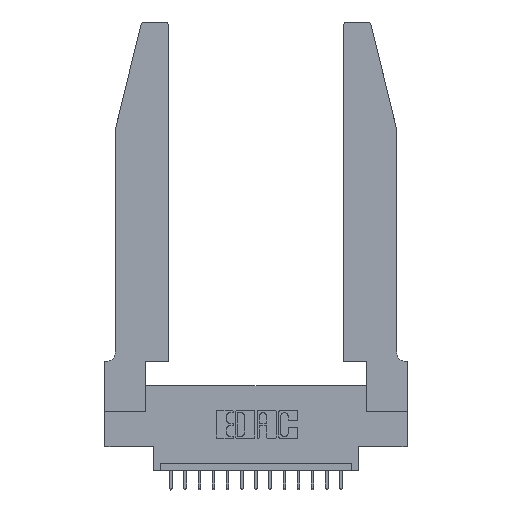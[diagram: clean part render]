
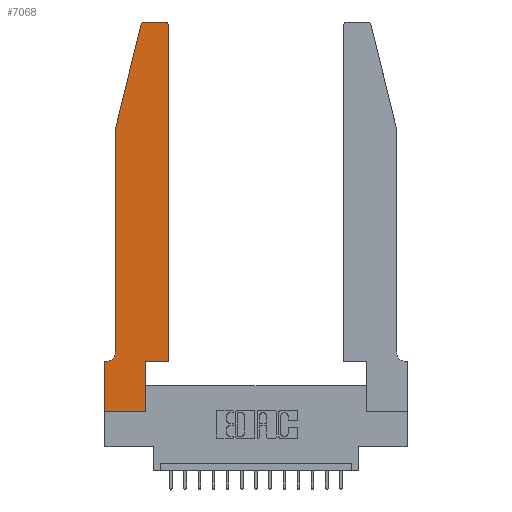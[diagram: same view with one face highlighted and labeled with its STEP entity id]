
A CAD part, top view. The second image highlights one B-rep face of the part: STEP entity #7068.
In plain terms, the highlighted planar face has unit normal (0, 0, 1).
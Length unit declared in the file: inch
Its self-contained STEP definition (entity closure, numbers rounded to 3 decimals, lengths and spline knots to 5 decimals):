
#320 = VERTEX_POINT ( 'NONE', #3296 ) ;
#523 = AXIS2_PLACEMENT_3D ( 'NONE', #9767, #8075, #13805 ) ;
#850 = VECTOR ( 'NONE', #7060, 39.37008 ) ;
#905 = VERTEX_POINT ( 'NONE', #1213 ) ;
#1090 = CIRCLE ( 'NONE', #15275, 0.03 ) ;
#1213 = CARTESIAN_POINT ( 'NONE',  ( 0.4205, 2.75, 0.37 ) ) ;
#1364 = CARTESIAN_POINT ( 'NONE',  ( 0.2865, 0.35, 0.37 ) ) ;
#1635 = VECTOR ( 'NONE', #4557, 39.37008 ) ;
#1688 = CARTESIAN_POINT ( 'NONE',  ( 0.4505, 0.35, 0.37 ) ) ;
#1705 = EDGE_CURVE ( 'NONE', #9627, #12850, #8957, .T. ) ;
#1714 = VERTEX_POINT ( 'NONE', #7247 ) ;
#1772 = DIRECTION ( 'NONE',  ( 0., 0., 1. ) ) ;
#1871 = EDGE_LOOP ( 'NONE', ( #9339, #7914, #3779, #16202, #6469, #6938, #16929, #7415, #16541, #7703, #12830, #9924 ) ) ;
#1991 = VERTEX_POINT ( 'NONE', #5051 ) ;
#2058 = CIRCLE ( 'NONE', #523, 0.07 ) ;
#2537 = DIRECTION ( 'NONE',  ( 0., 0., 1. ) ) ;
#3296 = CARTESIAN_POINT ( 'NONE',  ( 0.0755, 0.42, 0.37 ) ) ;
#3378 = EDGE_CURVE ( 'NONE', #17656, #9627, #1090, .T. ) ;
#3597 = CARTESIAN_POINT ( 'NONE',  ( 0., 0., 0.37 ) ) ;
#3779 = ORIENTED_EDGE ( 'NONE', *, *, #1705, .T. ) ;
#3914 = EDGE_CURVE ( 'NONE', #11699, #12863, #8164, .T. ) ;
#3939 = EDGE_CURVE ( 'NONE', #320, #15022, #2058, .T. ) ;
#3975 = DIRECTION ( 'NONE',  ( -1., 0., 0. ) ) ;
#4557 = DIRECTION ( 'NONE',  ( 1., 0., 0. ) ) ;
#4618 = EDGE_CURVE ( 'NONE', #12850, #320, #6096, .T. ) ;
#4737 = DIRECTION ( 'NONE',  ( 0., -1., 0. ) ) ;
#5051 = CARTESIAN_POINT ( 'NONE',  ( 0.4505, 2.72, 0.37 ) ) ;
#5394 = EDGE_CURVE ( 'NONE', #15397, #11699, #18429, .T. ) ;
#5614 = DIRECTION ( 'NONE',  ( 0., 1., 0. ) ) ;
#5744 = DIRECTION ( 'NONE',  ( 0., 0., 1. ) ) ;
#6096 = LINE ( 'NONE', #18585, #6936 ) ;
#6469 = ORIENTED_EDGE ( 'NONE', *, *, #3939, .T. ) ;
#6936 = VECTOR ( 'NONE', #11649, 39.37008 ) ;
#6938 = ORIENTED_EDGE ( 'NONE', *, *, #18564, .T. ) ;
#7060 = DIRECTION ( 'NONE',  ( 1., 0., 0. ) ) ;
#7068 = ADVANCED_FACE ( 'NONE', ( #10413 ), #16377, .T. ) ;
#7206 = VECTOR ( 'NONE', #5614, 39.37008 ) ;
#7247 = CARTESIAN_POINT ( 'NONE',  ( 0., 0.35, 0.37 ) ) ;
#7415 = ORIENTED_EDGE ( 'NONE', *, *, #5394, .T. ) ;
#7703 = ORIENTED_EDGE ( 'NONE', *, *, #15774, .T. ) ;
#7807 = CARTESIAN_POINT ( 'NONE',  ( 0.0055, 0.35, 0.37 ) ) ;
#7842 = CARTESIAN_POINT ( 'NONE',  ( 0.284, 2.75, 0.37 ) ) ;
#7914 = ORIENTED_EDGE ( 'NONE', *, *, #3378, .T. ) ;
#7948 = CARTESIAN_POINT ( 'NONE',  ( 0.25487, 2.72718, 0.37 ) ) ;
#8075 = DIRECTION ( 'NONE',  ( 0., 0., -1. ) ) ;
#8164 = LINE ( 'NONE', #15373, #7206 ) ;
#8316 = DIRECTION ( 'NONE',  ( -1., 0., 0. ) ) ;
#8335 = LINE ( 'NONE', #18026, #11259 ) ;
#8409 = LINE ( 'NONE', #17051, #10476 ) ;
#8413 = DIRECTION ( 'NONE',  ( 1., 0., 0. ) ) ;
#8957 = LINE ( 'NONE', #13075, #12099 ) ;
#8997 = VERTEX_POINT ( 'NONE', #9308 ) ;
#9222 = EDGE_CURVE ( 'NONE', #905, #17656, #8335, .T. ) ;
#9308 = CARTESIAN_POINT ( 'NONE',  ( 0.4505, 0.35, 0.37 ) ) ;
#9339 = ORIENTED_EDGE ( 'NONE', *, *, #9222, .T. ) ;
#9510 = VECTOR ( 'NONE', #4737, 39.37008 ) ;
#9627 = VERTEX_POINT ( 'NONE', #7948 ) ;
#9699 = CARTESIAN_POINT ( 'NONE',  ( 0., 0., 0.37 ) ) ;
#9767 = CARTESIAN_POINT ( 'NONE',  ( 0.0055, 0.42, 0.37 ) ) ;
#9911 = CARTESIAN_POINT ( 'NONE',  ( 0.2865, 0., 0.37 ) ) ;
#9924 = ORIENTED_EDGE ( 'NONE', *, *, #14533, .T. ) ;
#10084 = CIRCLE ( 'NONE', #12471, 0.03 ) ;
#10413 = FACE_OUTER_BOUND ( 'NONE', #1871, .T. ) ;
#10476 = VECTOR ( 'NONE', #8316, 39.37008 ) ;
#11259 = VECTOR ( 'NONE', #3975, 39.37008 ) ;
#11535 = DIRECTION ( 'NONE',  ( 1., 0., 0. ) ) ;
#11649 = DIRECTION ( 'NONE',  ( 0., -1., 0. ) ) ;
#11699 = VERTEX_POINT ( 'NONE', #9911 ) ;
#11739 = CARTESIAN_POINT ( 'NONE',  ( 0., 0., 0.37 ) ) ;
#12099 = VECTOR ( 'NONE', #14669, 39.37008 ) ;
#12471 = AXIS2_PLACEMENT_3D ( 'NONE', #16922, #5744, #12621 ) ;
#12621 = DIRECTION ( 'NONE',  ( 1., 0., 0. ) ) ;
#12649 = EDGE_CURVE ( 'NONE', #1714, #15397, #17537, .T. ) ;
#12830 = ORIENTED_EDGE ( 'NONE', *, *, #16238, .T. ) ;
#12850 = VERTEX_POINT ( 'NONE', #16479 ) ;
#12863 = VERTEX_POINT ( 'NONE', #1364 ) ;
#13075 = CARTESIAN_POINT ( 'NONE',  ( 0.0755, 2., 0.37 ) ) ;
#13805 = DIRECTION ( 'NONE',  ( -1., 0., 0. ) ) ;
#14533 = EDGE_CURVE ( 'NONE', #1991, #905, #10084, .T. ) ;
#14669 = DIRECTION ( 'NONE',  ( -0.239, -0.971, 0. ) ) ;
#14706 = CARTESIAN_POINT ( 'NONE',  ( 0., 0.35, 0.37 ) ) ;
#15022 = VERTEX_POINT ( 'NONE', #7807 ) ;
#15119 = CARTESIAN_POINT ( 'NONE',  ( 0.4505, 0.35, 0.37 ) ) ;
#15275 = AXIS2_PLACEMENT_3D ( 'NONE', #18563, #2537, #8413 ) ;
#15325 = AXIS2_PLACEMENT_3D ( 'NONE', #14706, #1772, #11535 ) ;
#15373 = CARTESIAN_POINT ( 'NONE',  ( 0.2865, 0.35, 0.37 ) ) ;
#15397 = VERTEX_POINT ( 'NONE', #3597 ) ;
#15774 = EDGE_CURVE ( 'NONE', #12863, #8997, #17448, .T. ) ;
#16202 = ORIENTED_EDGE ( 'NONE', *, *, #4618, .T. ) ;
#16238 = EDGE_CURVE ( 'NONE', #8997, #1991, #16705, .T. ) ;
#16337 = DIRECTION ( 'NONE',  ( 0., 1., 0. ) ) ;
#16377 = PLANE ( 'NONE',  #15325 ) ;
#16479 = CARTESIAN_POINT ( 'NONE',  ( 0.0755, 2., 0.37 ) ) ;
#16541 = ORIENTED_EDGE ( 'NONE', *, *, #3914, .T. ) ;
#16705 = LINE ( 'NONE', #15119, #17322 ) ;
#16922 = CARTESIAN_POINT ( 'NONE',  ( 0.4205, 2.72, 0.37 ) ) ;
#16929 = ORIENTED_EDGE ( 'NONE', *, *, #12649, .T. ) ;
#17051 = CARTESIAN_POINT ( 'NONE',  ( 0.0755, 0.35, 0.37 ) ) ;
#17322 = VECTOR ( 'NONE', #16337, 39.37008 ) ;
#17448 = LINE ( 'NONE', #1688, #1635 ) ;
#17537 = LINE ( 'NONE', #11739, #9510 ) ;
#17656 = VERTEX_POINT ( 'NONE', #7842 ) ;
#18026 = CARTESIAN_POINT ( 'NONE',  ( 0.2605, 2.75, 0.37 ) ) ;
#18429 = LINE ( 'NONE', #9699, #850 ) ;
#18563 = CARTESIAN_POINT ( 'NONE',  ( 0.284, 2.72, 0.37 ) ) ;
#18564 = EDGE_CURVE ( 'NONE', #15022, #1714, #8409, .T. ) ;
#18585 = CARTESIAN_POINT ( 'NONE',  ( 0.0755, 2., 0.37 ) ) ;
